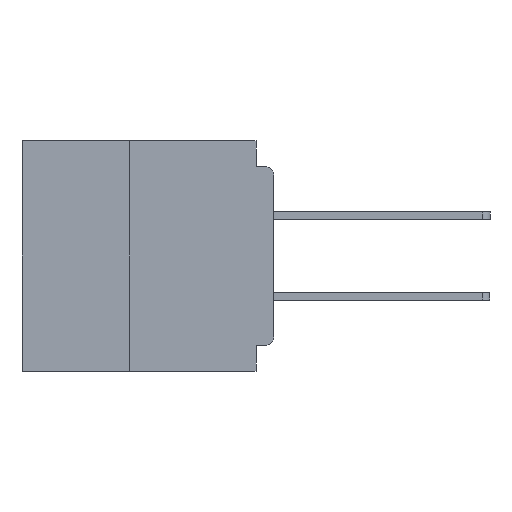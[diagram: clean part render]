
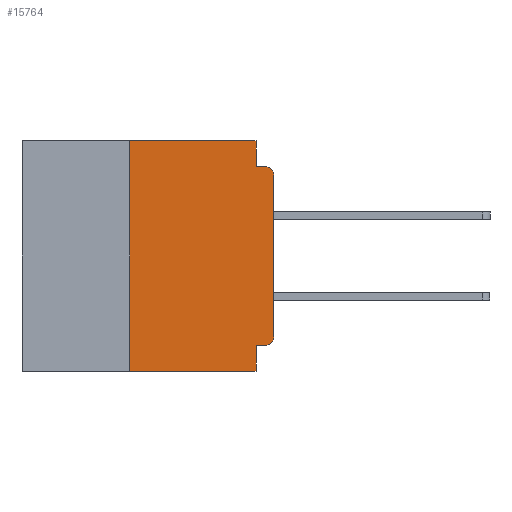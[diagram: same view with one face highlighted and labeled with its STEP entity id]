
A CAD part, left-side view. The second image highlights one B-rep face of the part: STEP entity #15764.
In plain terms, the highlighted planar face has unit normal (-1, 0, 0).
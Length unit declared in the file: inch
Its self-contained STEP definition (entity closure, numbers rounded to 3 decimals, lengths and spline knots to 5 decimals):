
#465 = LINE ( 'NONE', #54347, #10606 ) ;
#559 = LINE ( 'NONE', #12321, #45469 ) ;
#1456 = ORIENTED_EDGE ( 'NONE', *, *, #8398, .F. ) ;
#2512 = ORIENTED_EDGE ( 'NONE', *, *, #34171, .F. ) ;
#2875 = VERTEX_POINT ( 'NONE', #5786 ) ;
#3173 = CARTESIAN_POINT ( 'NONE',  ( 0., 0.031, -0.4 ) ) ;
#3430 = LINE ( 'NONE', #5260, #25144 ) ;
#3751 = DIRECTION ( 'NONE',  ( 0., 0., 1. ) ) ;
#4349 = ORIENTED_EDGE ( 'NONE', *, *, #26745, .F. ) ;
#4921 = FACE_OUTER_BOUND ( 'NONE', #27014, .T. ) ;
#5260 = CARTESIAN_POINT ( 'NONE',  ( 0., 0., 0. ) ) ;
#5381 = PLANE ( 'NONE',  #49405 ) ;
#5786 = CARTESIAN_POINT ( 'NONE',  ( 0., 0.015, -0.355 ) ) ;
#8107 = EDGE_CURVE ( 'NONE', #49172, #30898, #3430, .T. ) ;
#8398 = EDGE_CURVE ( 'NONE', #14785, #21255, #8762, .T. ) ;
#8762 = LINE ( 'NONE', #21058, #54487 ) ;
#9715 = DIRECTION ( 'NONE',  ( 0., 0., -1. ) ) ;
#10606 = VECTOR ( 'NONE', #23900, 39.37008 ) ;
#11466 = CARTESIAN_POINT ( 'NONE',  ( 0., 0.031, -0.355 ) ) ;
#12321 = CARTESIAN_POINT ( 'NONE',  ( 0., 0.437, 0. ) ) ;
#14035 = ORIENTED_EDGE ( 'NONE', *, *, #53861, .T. ) ;
#14785 = VERTEX_POINT ( 'NONE', #15538 ) ;
#15130 = VECTOR ( 'NONE', #36941, 39.37008 ) ;
#15538 = CARTESIAN_POINT ( 'NONE',  ( 0., 0.25, -0.4 ) ) ;
#15764 = ADVANCED_FACE ( 'NONE', ( #4921 ), #5381, .F. ) ;
#15903 = CARTESIAN_POINT ( 'NONE',  ( 0., 0., -0.34 ) ) ;
#16675 = AXIS2_PLACEMENT_3D ( 'NONE', #47240, #21177, #51616 ) ;
#16726 = DIRECTION ( 'NONE',  ( 0., -1., 0. ) ) ;
#17513 = EDGE_CURVE ( 'NONE', #2875, #49172, #51002, .T. ) ;
#17516 = CARTESIAN_POINT ( 'NONE',  ( 0., 0.031, 0. ) ) ;
#17994 = DIRECTION ( 'NONE',  ( 0., -1., 0. ) ) ;
#18414 = ORIENTED_EDGE ( 'NONE', *, *, #17513, .T. ) ;
#18443 = CARTESIAN_POINT ( 'NONE',  ( 0., 0., -0.06 ) ) ;
#18735 = CARTESIAN_POINT ( 'NONE',  ( 0., 0.015, -0.045 ) ) ;
#18837 = DIRECTION ( 'NONE',  ( -1., 0., 0. ) ) ;
#19050 = EDGE_CURVE ( 'NONE', #25501, #24239, #39303, .T. ) ;
#20879 = EDGE_CURVE ( 'NONE', #46411, #42263, #52065, .T. ) ;
#21058 = CARTESIAN_POINT ( 'NONE',  ( 0., 0.25, -0.4 ) ) ;
#21177 = DIRECTION ( 'NONE',  ( -1., 0., 0. ) ) ;
#21255 = VERTEX_POINT ( 'NONE', #34463 ) ;
#22568 = CIRCLE ( 'NONE', #40910, 0.015 ) ;
#23546 = VECTOR ( 'NONE', #17994, 39.37008 ) ;
#23900 = DIRECTION ( 'NONE',  ( 0., 1., 0. ) ) ;
#24205 = ORIENTED_EDGE ( 'NONE', *, *, #8107, .T. ) ;
#24239 = VERTEX_POINT ( 'NONE', #3173 ) ;
#25144 = VECTOR ( 'NONE', #35659, 39.37008 ) ;
#25501 = VERTEX_POINT ( 'NONE', #11466 ) ;
#26745 = EDGE_CURVE ( 'NONE', #2875, #25501, #465, .T. ) ;
#27014 = EDGE_LOOP ( 'NONE', ( #24205, #42256, #28970, #2512, #27857, #1456, #14035, #33463, #4349, #18414 ) ) ;
#27275 = DIRECTION ( 'NONE',  ( 0., -1., 0. ) ) ;
#27438 = DIRECTION ( 'NONE',  ( 0., 0., -1. ) ) ;
#27717 = VECTOR ( 'NONE', #27438, 39.37008 ) ;
#27857 = ORIENTED_EDGE ( 'NONE', *, *, #36823, .F. ) ;
#28970 = ORIENTED_EDGE ( 'NONE', *, *, #20879, .F. ) ;
#30898 = VERTEX_POINT ( 'NONE', #18443 ) ;
#31833 = CARTESIAN_POINT ( 'NONE',  ( 0., 0., -0.045 ) ) ;
#32389 = LINE ( 'NONE', #44081, #23546 ) ;
#32565 = CARTESIAN_POINT ( 'NONE',  ( 0., 0.031, 0. ) ) ;
#33463 = ORIENTED_EDGE ( 'NONE', *, *, #19050, .F. ) ;
#34171 = EDGE_CURVE ( 'NONE', #46624, #46411, #49865, .T. ) ;
#34463 = CARTESIAN_POINT ( 'NONE',  ( 0., 0.25, 0. ) ) ;
#34652 = EDGE_CURVE ( 'NONE', #30898, #42263, #22568, .T. ) ;
#35659 = DIRECTION ( 'NONE',  ( 0., 0., 1. ) ) ;
#35774 = DIRECTION ( 'NONE',  ( 1., 0., 0. ) ) ;
#36823 = EDGE_CURVE ( 'NONE', #21255, #46624, #559, .T. ) ;
#36941 = DIRECTION ( 'NONE',  ( 0., 0., -1. ) ) ;
#39303 = LINE ( 'NONE', #53534, #27717 ) ;
#40910 = AXIS2_PLACEMENT_3D ( 'NONE', #44912, #18837, #49256 ) ;
#42256 = ORIENTED_EDGE ( 'NONE', *, *, #34652, .T. ) ;
#42263 = VERTEX_POINT ( 'NONE', #18735 ) ;
#44081 = CARTESIAN_POINT ( 'NONE',  ( 0., 0.437, -0.4 ) ) ;
#44912 = CARTESIAN_POINT ( 'NONE',  ( 0., 0.015, -0.06 ) ) ;
#45469 = VECTOR ( 'NONE', #16726, 39.37008 ) ;
#46411 = VERTEX_POINT ( 'NONE', #46468 ) ;
#46468 = CARTESIAN_POINT ( 'NONE',  ( 0., 0.031, -0.045 ) ) ;
#46624 = VERTEX_POINT ( 'NONE', #17516 ) ;
#47240 = CARTESIAN_POINT ( 'NONE',  ( 0., 0.015, -0.34 ) ) ;
#49172 = VERTEX_POINT ( 'NONE', #15903 ) ;
#49256 = DIRECTION ( 'NONE',  ( 0., 0., -1. ) ) ;
#49302 = VECTOR ( 'NONE', #27275, 39.37008 ) ;
#49405 = AXIS2_PLACEMENT_3D ( 'NONE', #52961, #35774, #9715 ) ;
#49865 = LINE ( 'NONE', #32565, #15130 ) ;
#51002 = CIRCLE ( 'NONE', #16675, 0.015 ) ;
#51616 = DIRECTION ( 'NONE',  ( 0., 0., -1. ) ) ;
#52065 = LINE ( 'NONE', #31833, #49302 ) ;
#52961 = CARTESIAN_POINT ( 'NONE',  ( 0., 0.437, 0. ) ) ;
#53534 = CARTESIAN_POINT ( 'NONE',  ( 0., 0.031, -0.4 ) ) ;
#53861 = EDGE_CURVE ( 'NONE', #14785, #24239, #32389, .T. ) ;
#54347 = CARTESIAN_POINT ( 'NONE',  ( 0., 0., -0.355 ) ) ;
#54487 = VECTOR ( 'NONE', #3751, 39.37008 ) ;
